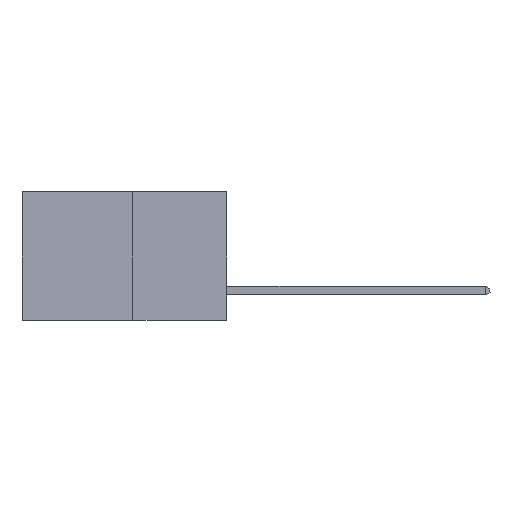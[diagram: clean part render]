
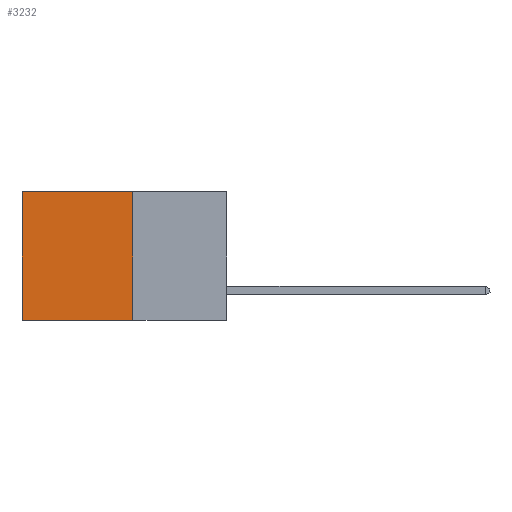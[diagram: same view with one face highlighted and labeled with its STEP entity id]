
A CAD part, left-side view. The second image highlights one B-rep face of the part: STEP entity #3232.
In plain terms, the highlighted planar face has unit normal (-1, 0, 0).
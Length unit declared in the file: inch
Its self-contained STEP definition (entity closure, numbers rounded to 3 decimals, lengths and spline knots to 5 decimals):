
#137 = PLANE ( 'NONE',  #6640 ) ;
#361 = VERTEX_POINT ( 'NONE', #1725 ) ;
#737 = CARTESIAN_POINT ( 'NONE',  ( 0.277, 0.27, -0.37 ) ) ;
#1293 = DIRECTION ( 'NONE',  ( 0., 1., 0. ) ) ;
#1553 = DIRECTION ( 'NONE',  ( 1., 0., 0. ) ) ;
#1725 = CARTESIAN_POINT ( 'NONE',  ( 0.277, 0.59, 0. ) ) ;
#2133 = ORIENTED_EDGE ( 'NONE', *, *, #6270, .T. ) ;
#2252 = CARTESIAN_POINT ( 'NONE',  ( 0.277, 0.27, -0.37 ) ) ;
#2392 = DIRECTION ( 'NONE',  ( 0., 0., -1. ) ) ;
#2520 = CARTESIAN_POINT ( 'NONE',  ( 0.277, 0.27, -0.37 ) ) ;
#2747 = VERTEX_POINT ( 'NONE', #10604 ) ;
#3232 = ADVANCED_FACE ( 'NONE', ( #3960 ), #137, .F. ) ;
#3237 = VECTOR ( 'NONE', #5410, 39.37008 ) ;
#3960 = FACE_OUTER_BOUND ( 'NONE', #11039, .T. ) ;
#4001 = VECTOR ( 'NONE', #7962, 39.37008 ) ;
#4077 = VERTEX_POINT ( 'NONE', #8833 ) ;
#4332 = DIRECTION ( 'NONE',  ( 0., 0., -1. ) ) ;
#4559 = LINE ( 'NONE', #737, #4001 ) ;
#5410 = DIRECTION ( 'NONE',  ( 0., 0., -1. ) ) ;
#5718 = CARTESIAN_POINT ( 'NONE',  ( 0.277, 0.27, -0.37 ) ) ;
#6270 = EDGE_CURVE ( 'NONE', #361, #2747, #8012, .T. ) ;
#6640 = AXIS2_PLACEMENT_3D ( 'NONE', #2252, #1553, #2392 ) ;
#6823 = LINE ( 'NONE', #2520, #8866 ) ;
#6843 = VERTEX_POINT ( 'NONE', #5718 ) ;
#7781 = ORIENTED_EDGE ( 'NONE', *, *, #9526, .F. ) ;
#7962 = DIRECTION ( 'NONE',  ( 0., 1., 0. ) ) ;
#8012 = LINE ( 'NONE', #9789, #3237 ) ;
#8048 = ORIENTED_EDGE ( 'NONE', *, *, #8970, .F. ) ;
#8833 = CARTESIAN_POINT ( 'NONE',  ( 0.277, 0.27, 0. ) ) ;
#8866 = VECTOR ( 'NONE', #4332, 39.37008 ) ;
#8970 = EDGE_CURVE ( 'NONE', #4077, #6843, #6823, .T. ) ;
#9354 = EDGE_CURVE ( 'NONE', #4077, #361, #9401, .T. ) ;
#9401 = LINE ( 'NONE', #10998, #11394 ) ;
#9526 = EDGE_CURVE ( 'NONE', #6843, #2747, #4559, .T. ) ;
#9789 = CARTESIAN_POINT ( 'NONE',  ( 0.277, 0.59, -0.37 ) ) ;
#10604 = CARTESIAN_POINT ( 'NONE',  ( 0.277, 0.59, -0.37 ) ) ;
#10998 = CARTESIAN_POINT ( 'NONE',  ( 0.277, 0.27, 0. ) ) ;
#11039 = EDGE_LOOP ( 'NONE', ( #2133, #7781, #8048, #11388 ) ) ;
#11388 = ORIENTED_EDGE ( 'NONE', *, *, #9354, .T. ) ;
#11394 = VECTOR ( 'NONE', #1293, 39.37008 ) ;
